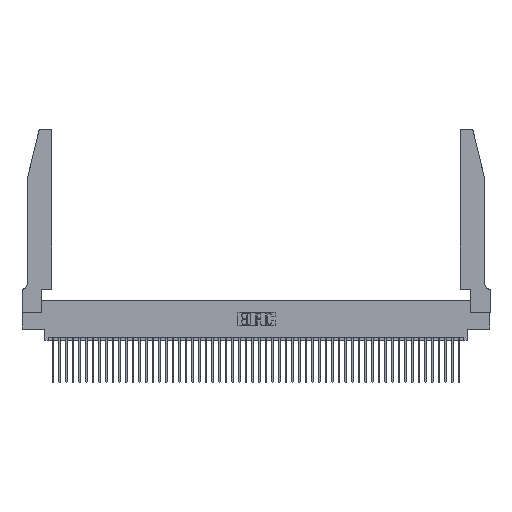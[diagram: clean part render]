
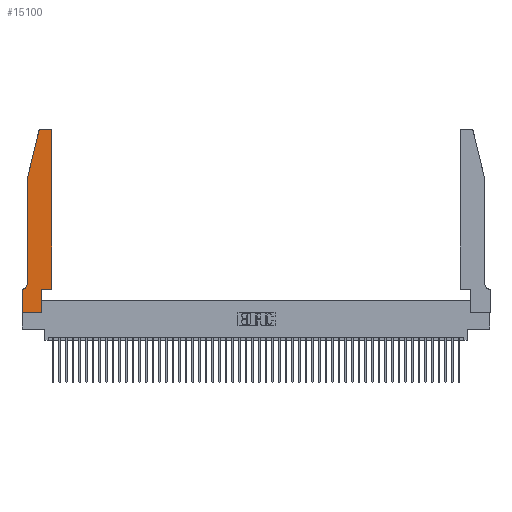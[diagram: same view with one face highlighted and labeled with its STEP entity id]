
A CAD part, top view. The second image highlights one B-rep face of the part: STEP entity #15100.
In plain terms, the highlighted planar face has unit normal (0, 0, 1).
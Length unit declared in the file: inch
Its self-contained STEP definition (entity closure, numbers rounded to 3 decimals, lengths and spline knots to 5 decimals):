
#205 = EDGE_CURVE ( 'NONE', #397, #36968, #19380, .T. ) ;
#397 = VERTEX_POINT ( 'NONE', #47514 ) ;
#886 = DIRECTION ( 'NONE',  ( 1., 0., 0. ) ) ;
#2329 = VERTEX_POINT ( 'NONE', #12792 ) ;
#3719 = EDGE_CURVE ( 'NONE', #20367, #14216, #6797, .T. ) ;
#3855 = FACE_OUTER_BOUND ( 'NONE', #27647, .T. ) ;
#3899 = ORIENTED_EDGE ( 'NONE', *, *, #19768, .T. ) ;
#4088 = ORIENTED_EDGE ( 'NONE', *, *, #22041, .T. ) ;
#4419 = VECTOR ( 'NONE', #48157, 39.37008 ) ;
#5600 = VECTOR ( 'NONE', #15502, 39.37008 ) ;
#5624 = DIRECTION ( 'NONE',  ( -1., 0., 0. ) ) ;
#5836 = DIRECTION ( 'NONE',  ( 0., 0., -1. ) ) ;
#6797 = LINE ( 'NONE', #11593, #5600 ) ;
#7187 = LINE ( 'NONE', #13855, #36658 ) ;
#7287 = LINE ( 'NONE', #13820, #19511 ) ;
#7739 = CARTESIAN_POINT ( 'NONE',  ( 0.4205, 2.75, 0.37 ) ) ;
#7839 = VERTEX_POINT ( 'NONE', #49607 ) ;
#8674 = VERTEX_POINT ( 'NONE', #18701 ) ;
#9012 = LINE ( 'NONE', #24664, #23071 ) ;
#11593 = CARTESIAN_POINT ( 'NONE',  ( 0.0755, 2., 0.37 ) ) ;
#12792 = CARTESIAN_POINT ( 'NONE',  ( 0., 0.35, 0.37 ) ) ;
#13087 = CARTESIAN_POINT ( 'NONE',  ( 0., 0., 0.37 ) ) ;
#13799 = EDGE_CURVE ( 'NONE', #2329, #37377, #29166, .T. ) ;
#13820 = CARTESIAN_POINT ( 'NONE',  ( 0.0755, 0.35, 0.37 ) ) ;
#13855 = CARTESIAN_POINT ( 'NONE',  ( 0.2605, 2.75, 0.37 ) ) ;
#13890 = VERTEX_POINT ( 'NONE', #7739 ) ;
#14216 = VERTEX_POINT ( 'NONE', #20927 ) ;
#14466 = CARTESIAN_POINT ( 'NONE',  ( 0.25487, 2.72718, 0.37 ) ) ;
#14561 = ORIENTED_EDGE ( 'NONE', *, *, #205, .T. ) ;
#14910 = CARTESIAN_POINT ( 'NONE',  ( 0.284, 2.72, 0.37 ) ) ;
#15100 = ADVANCED_FACE ( 'NONE', ( #3855 ), #31340, .T. ) ;
#15435 = DIRECTION ( 'NONE',  ( 1., 0., 0. ) ) ;
#15502 = DIRECTION ( 'NONE',  ( 0., -1., 0. ) ) ;
#15511 = CARTESIAN_POINT ( 'NONE',  ( 0.2865, 0.35, 0.37 ) ) ;
#15844 = CIRCLE ( 'NONE', #21265, 0.03 ) ;
#16228 = EDGE_CURVE ( 'NONE', #36968, #20367, #29586, .T. ) ;
#16408 = ORIENTED_EDGE ( 'NONE', *, *, #13799, .T. ) ;
#16528 = EDGE_CURVE ( 'NONE', #34592, #19654, #25276, .T. ) ;
#18324 = CARTESIAN_POINT ( 'NONE',  ( 0.4205, 2.72, 0.37 ) ) ;
#18701 = CARTESIAN_POINT ( 'NONE',  ( 0.0055, 0.35, 0.37 ) ) ;
#19011 = AXIS2_PLACEMENT_3D ( 'NONE', #26903, #27557, #46542 ) ;
#19380 = CIRCLE ( 'NONE', #20908, 0.03 ) ;
#19511 = VECTOR ( 'NONE', #5624, 39.37008 ) ;
#19654 = VERTEX_POINT ( 'NONE', #44588 ) ;
#19768 = EDGE_CURVE ( 'NONE', #8674, #2329, #7287, .T. ) ;
#20367 = VERTEX_POINT ( 'NONE', #32747 ) ;
#20908 = AXIS2_PLACEMENT_3D ( 'NONE', #14910, #22475, #42400 ) ;
#20927 = CARTESIAN_POINT ( 'NONE',  ( 0.0755, 0.42, 0.37 ) ) ;
#21232 = VECTOR ( 'NONE', #15435, 39.37008 ) ;
#21265 = AXIS2_PLACEMENT_3D ( 'NONE', #18324, #22592, #41525 ) ;
#21386 = DIRECTION ( 'NONE',  ( -1., 0., 0. ) ) ;
#22041 = EDGE_CURVE ( 'NONE', #37377, #7839, #50776, .T. ) ;
#22475 = DIRECTION ( 'NONE',  ( 0., 0., 1. ) ) ;
#22592 = DIRECTION ( 'NONE',  ( 0., 0., 1. ) ) ;
#22828 = VECTOR ( 'NONE', #48159, 39.37008 ) ;
#23003 = VECTOR ( 'NONE', #37799, 39.37008 ) ;
#23071 = VECTOR ( 'NONE', #886, 39.37008 ) ;
#23813 = EDGE_CURVE ( 'NONE', #7839, #40071, #35104, .T. ) ;
#24264 = ORIENTED_EDGE ( 'NONE', *, *, #27471, .T. ) ;
#24664 = CARTESIAN_POINT ( 'NONE',  ( 0.4505, 0.35, 0.37 ) ) ;
#25011 = CARTESIAN_POINT ( 'NONE',  ( 0.0055, 0.42, 0.37 ) ) ;
#25276 = LINE ( 'NONE', #47801, #4419 ) ;
#25366 = EDGE_CURVE ( 'NONE', #13890, #397, #7187, .T. ) ;
#26774 = ORIENTED_EDGE ( 'NONE', *, *, #16228, .T. ) ;
#26903 = CARTESIAN_POINT ( 'NONE',  ( 0., 0.35, 0.37 ) ) ;
#27129 = CARTESIAN_POINT ( 'NONE',  ( 0.0755, 2., 0.37 ) ) ;
#27471 = EDGE_CURVE ( 'NONE', #14216, #8674, #35140, .T. ) ;
#27557 = DIRECTION ( 'NONE',  ( 0., 0., 1. ) ) ;
#27647 = EDGE_LOOP ( 'NONE', ( #50825, #14561, #26774, #48900, #24264, #3899, #16408, #4088, #44004, #42743, #39369, #41809 ) ) ;
#29166 = LINE ( 'NONE', #45922, #23003 ) ;
#29586 = LINE ( 'NONE', #27129, #49350 ) ;
#31340 = PLANE ( 'NONE',  #19011 ) ;
#31672 = EDGE_CURVE ( 'NONE', #19654, #13890, #15844, .T. ) ;
#32075 = CARTESIAN_POINT ( 'NONE',  ( 0.2865, 0.35, 0.37 ) ) ;
#32747 = CARTESIAN_POINT ( 'NONE',  ( 0.0755, 2., 0.37 ) ) ;
#34592 = VERTEX_POINT ( 'NONE', #37564 ) ;
#35104 = LINE ( 'NONE', #32075, #22828 ) ;
#35140 = CIRCLE ( 'NONE', #46096, 0.07 ) ;
#36658 = VECTOR ( 'NONE', #21386, 39.37008 ) ;
#36968 = VERTEX_POINT ( 'NONE', #14466 ) ;
#37182 = DIRECTION ( 'NONE',  ( -1., 0., 0. ) ) ;
#37377 = VERTEX_POINT ( 'NONE', #13087 ) ;
#37564 = CARTESIAN_POINT ( 'NONE',  ( 0.4505, 0.35, 0.37 ) ) ;
#37799 = DIRECTION ( 'NONE',  ( 0., -1., 0. ) ) ;
#38173 = DIRECTION ( 'NONE',  ( -0.239, -0.971, 0. ) ) ;
#38931 = EDGE_CURVE ( 'NONE', #40071, #34592, #9012, .T. ) ;
#39369 = ORIENTED_EDGE ( 'NONE', *, *, #16528, .T. ) ;
#40071 = VERTEX_POINT ( 'NONE', #15511 ) ;
#41525 = DIRECTION ( 'NONE',  ( 1., 0., 0. ) ) ;
#41809 = ORIENTED_EDGE ( 'NONE', *, *, #31672, .T. ) ;
#42400 = DIRECTION ( 'NONE',  ( 1., 0., 0. ) ) ;
#42743 = ORIENTED_EDGE ( 'NONE', *, *, #38931, .T. ) ;
#42767 = CARTESIAN_POINT ( 'NONE',  ( 0., 0., 0.37 ) ) ;
#44004 = ORIENTED_EDGE ( 'NONE', *, *, #23813, .T. ) ;
#44588 = CARTESIAN_POINT ( 'NONE',  ( 0.4505, 2.72, 0.37 ) ) ;
#45922 = CARTESIAN_POINT ( 'NONE',  ( 0., 0., 0.37 ) ) ;
#46096 = AXIS2_PLACEMENT_3D ( 'NONE', #25011, #5836, #37182 ) ;
#46542 = DIRECTION ( 'NONE',  ( 1., 0., 0. ) ) ;
#47514 = CARTESIAN_POINT ( 'NONE',  ( 0.284, 2.75, 0.37 ) ) ;
#47801 = CARTESIAN_POINT ( 'NONE',  ( 0.4505, 0.35, 0.37 ) ) ;
#48157 = DIRECTION ( 'NONE',  ( 0., 1., 0. ) ) ;
#48159 = DIRECTION ( 'NONE',  ( 0., 1., 0. ) ) ;
#48900 = ORIENTED_EDGE ( 'NONE', *, *, #3719, .T. ) ;
#49350 = VECTOR ( 'NONE', #38173, 39.37008 ) ;
#49607 = CARTESIAN_POINT ( 'NONE',  ( 0.2865, 0., 0.37 ) ) ;
#50776 = LINE ( 'NONE', #42767, #21232 ) ;
#50825 = ORIENTED_EDGE ( 'NONE', *, *, #25366, .T. ) ;
